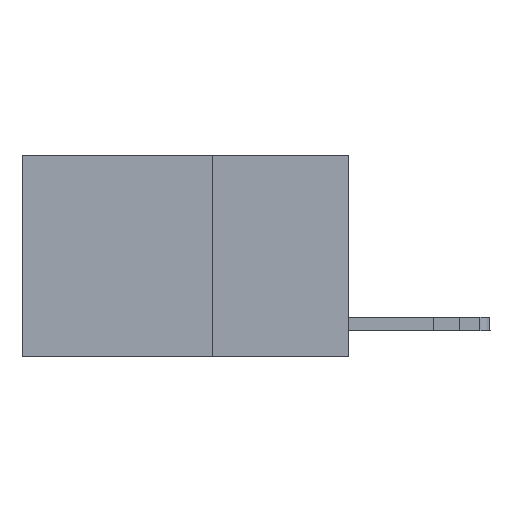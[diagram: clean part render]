
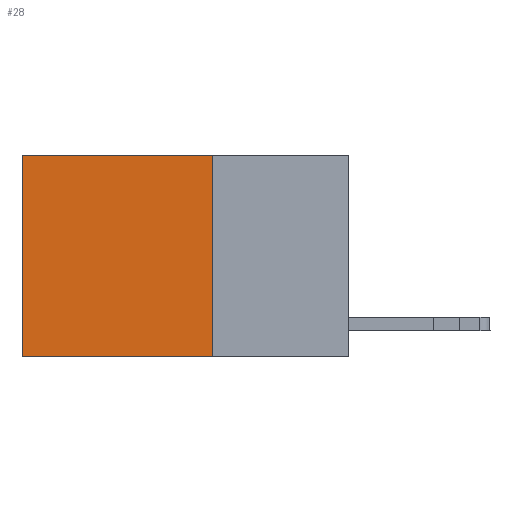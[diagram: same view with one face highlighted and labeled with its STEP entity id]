
A CAD part, left-side view. The second image highlights one B-rep face of the part: STEP entity #28.
In plain terms, the highlighted planar face has unit normal (-1, 0, 0).
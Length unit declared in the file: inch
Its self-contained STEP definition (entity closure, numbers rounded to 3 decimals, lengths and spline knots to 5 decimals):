
#28 = ADVANCED_FACE ( 'NONE', ( #2540 ), #9831, .F. ) ;
#1254 = VERTEX_POINT ( 'NONE', #10615 ) ;
#1400 = EDGE_LOOP ( 'NONE', ( #9680, #12017, #4717, #2771 ) ) ;
#1972 = CARTESIAN_POINT ( 'NONE',  ( 0.2625, 0.6, 0. ) ) ;
#2411 = DIRECTION ( 'NONE',  ( 1., 0., 0. ) ) ;
#2540 = FACE_OUTER_BOUND ( 'NONE', #1400, .T. ) ;
#2743 = VERTEX_POINT ( 'NONE', #1972 ) ;
#2771 = ORIENTED_EDGE ( 'NONE', *, *, #12490, .T. ) ;
#4200 = CARTESIAN_POINT ( 'NONE',  ( 0.2625, 0.6, 0. ) ) ;
#4233 = EDGE_CURVE ( 'NONE', #5174, #1254, #7632, .T. ) ;
#4260 = CARTESIAN_POINT ( 'NONE',  ( 0.2625, 0.25, -0.37 ) ) ;
#4354 = DIRECTION ( 'NONE',  ( 0., 1., 0. ) ) ;
#4717 = ORIENTED_EDGE ( 'NONE', *, *, #4957, .F. ) ;
#4851 = LINE ( 'NONE', #11023, #9848 ) ;
#4895 = VECTOR ( 'NONE', #4354, 39.37008 ) ;
#4957 = EDGE_CURVE ( 'NONE', #5197, #5174, #5585, .T. ) ;
#4963 = LINE ( 'NONE', #4200, #10225 ) ;
#5174 = VERTEX_POINT ( 'NONE', #10417 ) ;
#5197 = VERTEX_POINT ( 'NONE', #10285 ) ;
#5342 = AXIS2_PLACEMENT_3D ( 'NONE', #6485, #2411, #11044 ) ;
#5585 = LINE ( 'NONE', #9930, #7944 ) ;
#6485 = CARTESIAN_POINT ( 'NONE',  ( 0.2625, 0.25, 0. ) ) ;
#7233 = DIRECTION ( 'NONE',  ( 0., 1., 0. ) ) ;
#7632 = LINE ( 'NONE', #4260, #4895 ) ;
#7738 = DIRECTION ( 'NONE',  ( 0., 0., -1. ) ) ;
#7944 = VECTOR ( 'NONE', #7738, 39.37008 ) ;
#9680 = ORIENTED_EDGE ( 'NONE', *, *, #10145, .T. ) ;
#9831 = PLANE ( 'NONE',  #5342 ) ;
#9848 = VECTOR ( 'NONE', #7233, 39.37008 ) ;
#9930 = CARTESIAN_POINT ( 'NONE',  ( 0.2625, 0.25, 0. ) ) ;
#10145 = EDGE_CURVE ( 'NONE', #2743, #1254, #4963, .T. ) ;
#10225 = VECTOR ( 'NONE', #11109, 39.37008 ) ;
#10285 = CARTESIAN_POINT ( 'NONE',  ( 0.2625, 0.25, 0. ) ) ;
#10417 = CARTESIAN_POINT ( 'NONE',  ( 0.2625, 0.25, -0.37 ) ) ;
#10615 = CARTESIAN_POINT ( 'NONE',  ( 0.2625, 0.6, -0.37 ) ) ;
#11023 = CARTESIAN_POINT ( 'NONE',  ( 0.2625, 0.25, 0. ) ) ;
#11044 = DIRECTION ( 'NONE',  ( 0., 0., -1. ) ) ;
#11109 = DIRECTION ( 'NONE',  ( 0., 0., -1. ) ) ;
#12017 = ORIENTED_EDGE ( 'NONE', *, *, #4233, .F. ) ;
#12490 = EDGE_CURVE ( 'NONE', #5197, #2743, #4851, .T. ) ;
